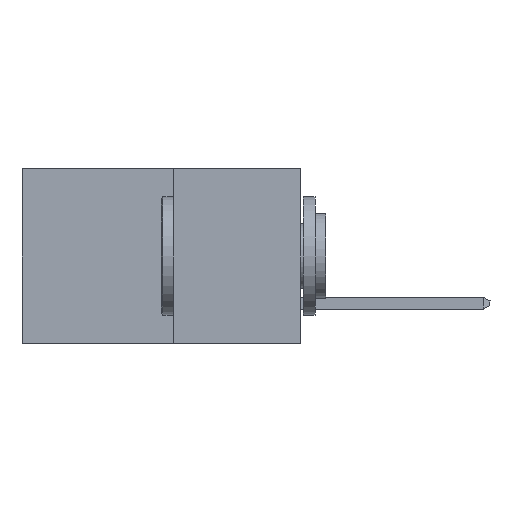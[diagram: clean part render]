
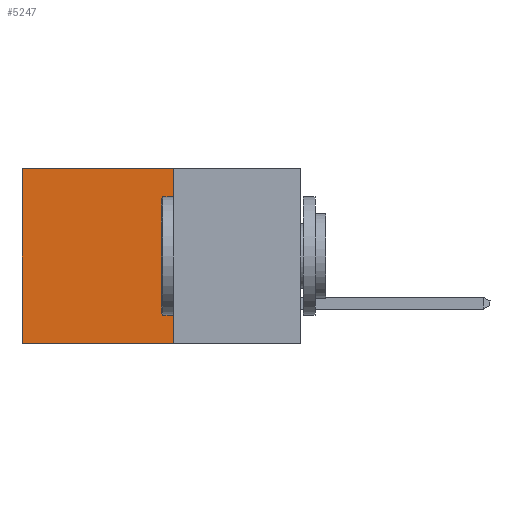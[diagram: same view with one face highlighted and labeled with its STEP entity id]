
A CAD part, left-side view. The second image highlights one B-rep face of the part: STEP entity #5247.
In plain terms, the highlighted planar face has unit normal (-1, 0, 0).
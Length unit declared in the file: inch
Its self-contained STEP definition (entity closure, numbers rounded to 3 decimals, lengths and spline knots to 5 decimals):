
#276 = CARTESIAN_POINT ( 'NONE',  ( 0.277, 0.27, -0.37 ) ) ;
#304 = LINE ( 'NONE', #5025, #28530 ) ;
#655 = CARTESIAN_POINT ( 'NONE',  ( 0.277, 0.59, -0.37 ) ) ;
#836 = LINE ( 'NONE', #24684, #24433 ) ;
#857 = DIRECTION ( 'NONE',  ( 0., 0., -1. ) ) ;
#2964 = EDGE_CURVE ( 'NONE', #18359, #14586, #16472, .T. ) ;
#3923 = ORIENTED_EDGE ( 'NONE', *, *, #18239, .F. ) ;
#4606 = CARTESIAN_POINT ( 'NONE',  ( 0.277, 0.59, 0. ) ) ;
#5025 = CARTESIAN_POINT ( 'NONE',  ( 0.277, 0.27, 0. ) ) ;
#5247 = ADVANCED_FACE ( 'NONE', ( #16470 ), #7179, .F. ) ;
#5824 = CARTESIAN_POINT ( 'NONE',  ( 0.277, 0.27, 0. ) ) ;
#6010 = CARTESIAN_POINT ( 'NONE',  ( 0.277, 0.27, -0.37 ) ) ;
#6539 = EDGE_CURVE ( 'NONE', #20939, #18359, #304, .T. ) ;
#7179 = PLANE ( 'NONE',  #27314 ) ;
#7387 = CARTESIAN_POINT ( 'NONE',  ( 0.277, 0.27, -0.37 ) ) ;
#9457 = DIRECTION ( 'NONE',  ( 1., 0., 0. ) ) ;
#9700 = VERTEX_POINT ( 'NONE', #6010 ) ;
#10998 = DIRECTION ( 'NONE',  ( 0., 1., 0. ) ) ;
#13903 = EDGE_LOOP ( 'NONE', ( #22390, #3923, #29367, #22787 ) ) ;
#14586 = VERTEX_POINT ( 'NONE', #23206 ) ;
#16187 = VECTOR ( 'NONE', #21086, 39.37008 ) ;
#16470 = FACE_OUTER_BOUND ( 'NONE', #13903, .T. ) ;
#16472 = LINE ( 'NONE', #655, #27888 ) ;
#18239 = EDGE_CURVE ( 'NONE', #9700, #14586, #836, .T. ) ;
#18359 = VERTEX_POINT ( 'NONE', #4606 ) ;
#19356 = EDGE_CURVE ( 'NONE', #20939, #9700, #22267, .T. ) ;
#20939 = VERTEX_POINT ( 'NONE', #5824 ) ;
#21086 = DIRECTION ( 'NONE',  ( 0., 0., -1. ) ) ;
#22267 = LINE ( 'NONE', #7387, #16187 ) ;
#22390 = ORIENTED_EDGE ( 'NONE', *, *, #2964, .T. ) ;
#22787 = ORIENTED_EDGE ( 'NONE', *, *, #6539, .T. ) ;
#23206 = CARTESIAN_POINT ( 'NONE',  ( 0.277, 0.59, -0.37 ) ) ;
#23311 = DIRECTION ( 'NONE',  ( 0., 1., 0. ) ) ;
#24433 = VECTOR ( 'NONE', #10998, 39.37008 ) ;
#24684 = CARTESIAN_POINT ( 'NONE',  ( 0.277, 0.27, -0.37 ) ) ;
#25451 = DIRECTION ( 'NONE',  ( 0., 0., -1. ) ) ;
#27314 = AXIS2_PLACEMENT_3D ( 'NONE', #276, #9457, #25451 ) ;
#27888 = VECTOR ( 'NONE', #857, 39.37008 ) ;
#28530 = VECTOR ( 'NONE', #23311, 39.37008 ) ;
#29367 = ORIENTED_EDGE ( 'NONE', *, *, #19356, .F. ) ;
